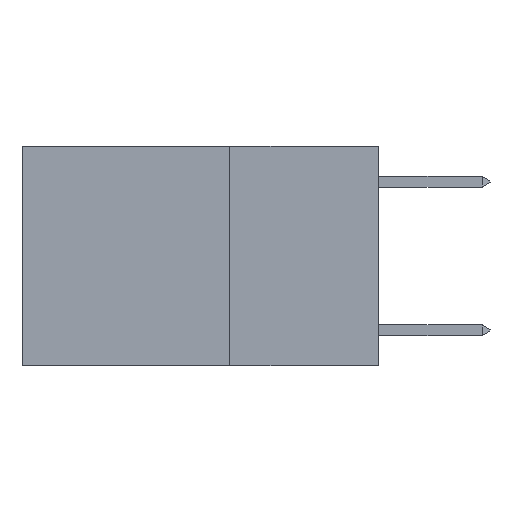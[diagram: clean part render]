
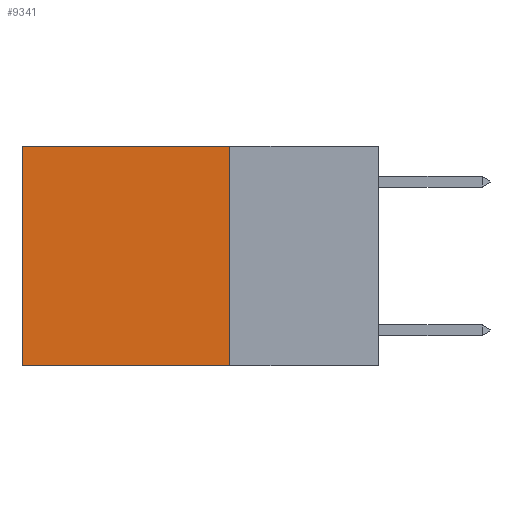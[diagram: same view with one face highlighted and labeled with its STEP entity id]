
A CAD part, left-side view. The second image highlights one B-rep face of the part: STEP entity #9341.
In plain terms, the highlighted planar face has unit normal (-1, 0, 0).
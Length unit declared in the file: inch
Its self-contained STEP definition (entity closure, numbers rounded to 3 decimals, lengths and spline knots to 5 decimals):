
#297 = VECTOR ( 'NONE', #2706, 39.37008 ) ;
#759 = CARTESIAN_POINT ( 'NONE',  ( 0.2625, 0.25, 0. ) ) ;
#888 = EDGE_CURVE ( 'NONE', #1297, #1594, #5943, .T. ) ;
#1184 = PLANE ( 'NONE',  #4455 ) ;
#1297 = VERTEX_POINT ( 'NONE', #759 ) ;
#1399 = CARTESIAN_POINT ( 'NONE',  ( 0.2625, 0.25, -0.37 ) ) ;
#1594 = VERTEX_POINT ( 'NONE', #12488 ) ;
#2241 = CARTESIAN_POINT ( 'NONE',  ( 0.2625, 0.25, 0. ) ) ;
#2255 = VECTOR ( 'NONE', #12915, 39.37008 ) ;
#2642 = LINE ( 'NONE', #7742, #297 ) ;
#2706 = DIRECTION ( 'NONE',  ( 0., 0., -1. ) ) ;
#3378 = DIRECTION ( 'NONE',  ( 0., 1., 0. ) ) ;
#3734 = ORIENTED_EDGE ( 'NONE', *, *, #12316, .T. ) ;
#4455 = AXIS2_PLACEMENT_3D ( 'NONE', #2241, #10797, #11234 ) ;
#5070 = ORIENTED_EDGE ( 'NONE', *, *, #10662, .F. ) ;
#5427 = VERTEX_POINT ( 'NONE', #5817 ) ;
#5735 = DIRECTION ( 'NONE',  ( 0., 0., -1. ) ) ;
#5817 = CARTESIAN_POINT ( 'NONE',  ( 0.2625, 0.25, -0.37 ) ) ;
#5943 = LINE ( 'NONE', #8956, #2255 ) ;
#6521 = CARTESIAN_POINT ( 'NONE',  ( 0.2625, 0.6, -0.37 ) ) ;
#6662 = CARTESIAN_POINT ( 'NONE',  ( 0.2625, 0.25, 0. ) ) ;
#7418 = EDGE_LOOP ( 'NONE', ( #3734, #5070, #11207, #10436 ) ) ;
#7742 = CARTESIAN_POINT ( 'NONE',  ( 0.2625, 0.6, 0. ) ) ;
#7846 = VECTOR ( 'NONE', #3378, 39.37008 ) ;
#7879 = FACE_OUTER_BOUND ( 'NONE', #7418, .T. ) ;
#8782 = VERTEX_POINT ( 'NONE', #6521 ) ;
#8956 = CARTESIAN_POINT ( 'NONE',  ( 0.2625, 0.25, 0. ) ) ;
#9320 = LINE ( 'NONE', #1399, #7846 ) ;
#9341 = ADVANCED_FACE ( 'NONE', ( #7879 ), #1184, .F. ) ;
#10436 = ORIENTED_EDGE ( 'NONE', *, *, #888, .T. ) ;
#10662 = EDGE_CURVE ( 'NONE', #5427, #8782, #9320, .T. ) ;
#10701 = LINE ( 'NONE', #6662, #12207 ) ;
#10797 = DIRECTION ( 'NONE',  ( 1., 0., 0. ) ) ;
#11207 = ORIENTED_EDGE ( 'NONE', *, *, #12636, .F. ) ;
#11234 = DIRECTION ( 'NONE',  ( 0., 0., -1. ) ) ;
#12207 = VECTOR ( 'NONE', #5735, 39.37008 ) ;
#12316 = EDGE_CURVE ( 'NONE', #1594, #8782, #2642, .T. ) ;
#12488 = CARTESIAN_POINT ( 'NONE',  ( 0.2625, 0.6, 0. ) ) ;
#12636 = EDGE_CURVE ( 'NONE', #1297, #5427, #10701, .T. ) ;
#12915 = DIRECTION ( 'NONE',  ( 0., 1., 0. ) ) ;
